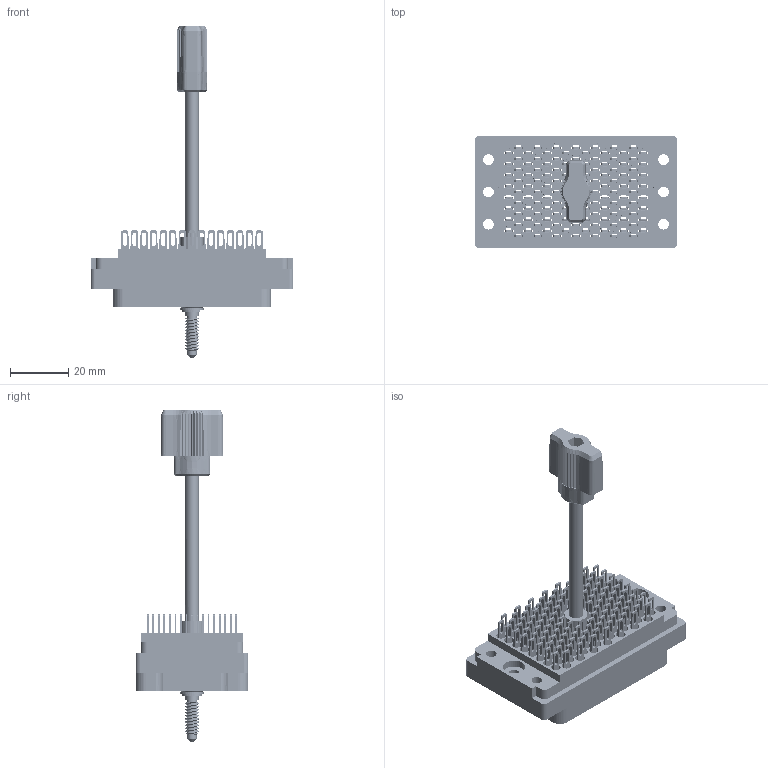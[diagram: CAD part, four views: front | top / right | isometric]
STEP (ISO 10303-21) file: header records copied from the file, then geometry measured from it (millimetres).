
FILE_DESCRIPTION (( 'STEP AP203' ), '1' );
FILE_NAME ('516-120-500-305.STEP', '2020-03-11T02:32:59', ( '' ), ( '' ), 'SwSTEP 2.0', 'SolidWorks 2016', '' );
FILE_SCHEMA (( 'CONFIG_CONTROL_DESIGN' ));
Length unit declared in the file: inch
Products named in the file (10): Actuating Screw Assy 090-120; 516-251-095-100; Grub Screw; 516-254-091-109; 516-120-500-305; 516-253-095-100; 516-292-001_500 Contact; 516-253-190-107; 516 Plug Insulator_120; 516-250-091-111
Assembly tree (129 placements, depth 3):
  516-120-500-305
    516 Plug Insulator_120
    516-292-001_500 Contact  x120
    Actuating Screw Assy 090-120
      516-251-095-100
      516-254-091-109
      516-253-095-100  x2
      516-253-190-107
      516-250-091-111
      Grub Screw
Bounding box: 69.85 x 38.73 x 114.34 mm (x, y, z)
Volume: 28730.8 mm3; surface area: 53102.6 mm2
Topology: 128 solids, 128 shells, 11801 faces, 34251 edges, 22726 vertices
Faces by surface type: plane 7071, cylinder 3931, bspline 737, cone 62
Entity records: 103482 total; most frequent: CARTESIAN_POINT 23862, ORIENTED_EDGE 16118, DIRECTION 15461, EDGE_CURVE 8059, VECTOR 5917, LINE 5917, VERTEX_POINT 5344, AXIS2_PLACEMENT_3D 4772
